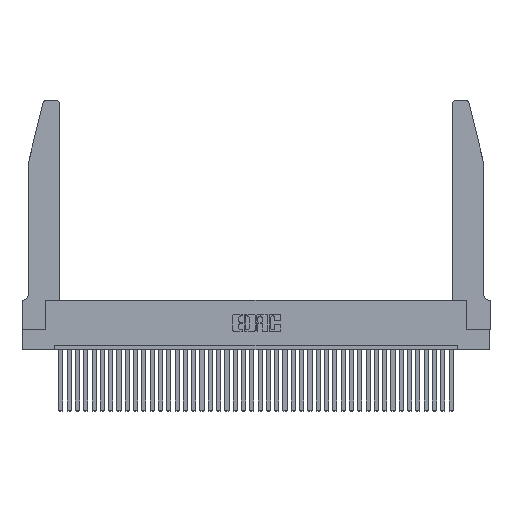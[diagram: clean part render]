
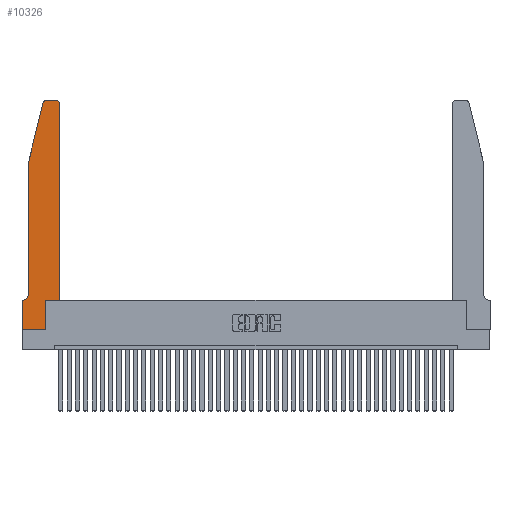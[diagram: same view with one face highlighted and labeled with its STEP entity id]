
A CAD part, top view. The second image highlights one B-rep face of the part: STEP entity #10326.
In plain terms, the highlighted planar face has unit normal (0, 0, 1).
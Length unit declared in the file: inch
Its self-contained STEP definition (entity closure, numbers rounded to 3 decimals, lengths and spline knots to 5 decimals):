
#589 = VERTEX_POINT ( 'NONE', #13890 ) ;
#645 = EDGE_CURVE ( 'NONE', #35161, #6498, #15695, .T. ) ;
#1042 = DIRECTION ( 'NONE',  ( 0., 1., 0. ) ) ;
#1490 = CARTESIAN_POINT ( 'NONE',  ( 0.4205, 2.75, 0.37 ) ) ;
#2235 = ORIENTED_EDGE ( 'NONE', *, *, #22283, .T. ) ;
#3429 = CIRCLE ( 'NONE', #34982, 0.03 ) ;
#4097 = VECTOR ( 'NONE', #7911, 39.37008 ) ;
#4209 = CARTESIAN_POINT ( 'NONE',  ( 0.4505, 0.35, 0.37 ) ) ;
#4305 = CARTESIAN_POINT ( 'NONE',  ( 0.0755, 2., 0.37 ) ) ;
#4544 = VECTOR ( 'NONE', #25176, 39.37008 ) ;
#4621 = LINE ( 'NONE', #5936, #9908 ) ;
#4705 = DIRECTION ( 'NONE',  ( 0., -1., 0. ) ) ;
#4820 = CARTESIAN_POINT ( 'NONE',  ( 0.2865, 0.35, 0.37 ) ) ;
#5300 = EDGE_CURVE ( 'NONE', #589, #15659, #29357, .T. ) ;
#5936 = CARTESIAN_POINT ( 'NONE',  ( 0.2605, 2.75, 0.37 ) ) ;
#6114 = CARTESIAN_POINT ( 'NONE',  ( 0., 0., 0.37 ) ) ;
#6163 = CARTESIAN_POINT ( 'NONE',  ( 0.284, 2.75, 0.37 ) ) ;
#6392 = EDGE_CURVE ( 'NONE', #20870, #37852, #35029, .T. ) ;
#6498 = VERTEX_POINT ( 'NONE', #14295 ) ;
#6623 = VECTOR ( 'NONE', #18837, 39.37008 ) ;
#7006 = VECTOR ( 'NONE', #1042, 39.37008 ) ;
#7141 = DIRECTION ( 'NONE',  ( 1., 0., 0. ) ) ;
#7183 = CARTESIAN_POINT ( 'NONE',  ( 0.0755, 0.35, 0.37 ) ) ;
#7505 = CARTESIAN_POINT ( 'NONE',  ( 0.0755, 2., 0.37 ) ) ;
#7640 = DIRECTION ( 'NONE',  ( -0.239, -0.971, 0. ) ) ;
#7911 = DIRECTION ( 'NONE',  ( 0., -1., 0. ) ) ;
#7989 = DIRECTION ( 'NONE',  ( 1., 0., 0. ) ) ;
#8179 = CARTESIAN_POINT ( 'NONE',  ( 0., 0.35, 0.37 ) ) ;
#8869 = EDGE_CURVE ( 'NONE', #38321, #37505, #3429, .T. ) ;
#8911 = DIRECTION ( 'NONE',  ( -1., 0., 0. ) ) ;
#9540 = LINE ( 'NONE', #6114, #6623 ) ;
#9835 = ORIENTED_EDGE ( 'NONE', *, *, #6392, .T. ) ;
#9908 = VECTOR ( 'NONE', #8911, 39.37008 ) ;
#10326 = ADVANCED_FACE ( 'NONE', ( #18311 ), #38948, .T. ) ;
#11363 = ORIENTED_EDGE ( 'NONE', *, *, #24480, .T. ) ;
#11389 = CARTESIAN_POINT ( 'NONE',  ( 0., 0., 0.37 ) ) ;
#11630 = CARTESIAN_POINT ( 'NONE',  ( 0., 0., 0.37 ) ) ;
#12373 = DIRECTION ( 'NONE',  ( -1., 0., 0. ) ) ;
#13304 = VECTOR ( 'NONE', #4705, 39.37008 ) ;
#13830 = CARTESIAN_POINT ( 'NONE',  ( 0.4505, 2.72, 0.37 ) ) ;
#13890 = CARTESIAN_POINT ( 'NONE',  ( 0.0755, 0.42, 0.37 ) ) ;
#14129 = DIRECTION ( 'NONE',  ( 1., 0., 0. ) ) ;
#14295 = CARTESIAN_POINT ( 'NONE',  ( 0.4505, 0.35, 0.37 ) ) ;
#14381 = DIRECTION ( 'NONE',  ( 0., 0., 1. ) ) ;
#15659 = VERTEX_POINT ( 'NONE', #33904 ) ;
#15695 = LINE ( 'NONE', #4209, #39764 ) ;
#16144 = CARTESIAN_POINT ( 'NONE',  ( 0.2865, 0.35, 0.37 ) ) ;
#17156 = DIRECTION ( 'NONE',  ( 1., 0., 0. ) ) ;
#17570 = ORIENTED_EDGE ( 'NONE', *, *, #8869, .T. ) ;
#17880 = ORIENTED_EDGE ( 'NONE', *, *, #645, .T. ) ;
#18311 = FACE_OUTER_BOUND ( 'NONE', #35953, .T. ) ;
#18477 = AXIS2_PLACEMENT_3D ( 'NONE', #8179, #14381, #14129 ) ;
#18837 = DIRECTION ( 'NONE',  ( 1., 0., 0. ) ) ;
#19329 = EDGE_CURVE ( 'NONE', #37852, #38331, #9540, .T. ) ;
#19630 = DIRECTION ( 'NONE',  ( -1., 0., 0. ) ) ;
#19661 = ORIENTED_EDGE ( 'NONE', *, *, #22123, .T. ) ;
#19864 = CARTESIAN_POINT ( 'NONE',  ( 0., 0.35, 0.37 ) ) ;
#20043 = LINE ( 'NONE', #34841, #7006 ) ;
#20467 = VECTOR ( 'NONE', #7640, 39.37008 ) ;
#20529 = DIRECTION ( 'NONE',  ( 0., 0., 1. ) ) ;
#20870 = VERTEX_POINT ( 'NONE', #19864 ) ;
#21017 = EDGE_CURVE ( 'NONE', #28596, #33190, #23920, .T. ) ;
#21242 = EDGE_CURVE ( 'NONE', #6498, #28596, #20043, .T. ) ;
#21863 = CARTESIAN_POINT ( 'NONE',  ( 0.0055, 0.42, 0.37 ) ) ;
#21864 = CARTESIAN_POINT ( 'NONE',  ( 0.0755, 2., 0.37 ) ) ;
#22123 = EDGE_CURVE ( 'NONE', #26755, #589, #32594, .T. ) ;
#22283 = EDGE_CURVE ( 'NONE', #37505, #26755, #29636, .T. ) ;
#23566 = DIRECTION ( 'NONE',  ( 0., 0., 1. ) ) ;
#23688 = CARTESIAN_POINT ( 'NONE',  ( 0.284, 2.72, 0.37 ) ) ;
#23920 = CIRCLE ( 'NONE', #24171, 0.03 ) ;
#24171 = AXIS2_PLACEMENT_3D ( 'NONE', #32954, #20529, #17156 ) ;
#24480 = EDGE_CURVE ( 'NONE', #15659, #20870, #31365, .T. ) ;
#24566 = DIRECTION ( 'NONE',  ( 0., 0., -1. ) ) ;
#25176 = DIRECTION ( 'NONE',  ( 0., 1., 0. ) ) ;
#26254 = ORIENTED_EDGE ( 'NONE', *, *, #30677, .T. ) ;
#26593 = EDGE_CURVE ( 'NONE', #38331, #35161, #30578, .T. ) ;
#26755 = VERTEX_POINT ( 'NONE', #21864 ) ;
#27018 = ORIENTED_EDGE ( 'NONE', *, *, #21242, .T. ) ;
#28596 = VERTEX_POINT ( 'NONE', #13830 ) ;
#28714 = ORIENTED_EDGE ( 'NONE', *, *, #21017, .T. ) ;
#29357 = CIRCLE ( 'NONE', #31567, 0.07 ) ;
#29636 = LINE ( 'NONE', #7505, #20467 ) ;
#29761 = ORIENTED_EDGE ( 'NONE', *, *, #19329, .T. ) ;
#30578 = LINE ( 'NONE', #16144, #4544 ) ;
#30677 = EDGE_CURVE ( 'NONE', #33190, #38321, #4621, .T. ) ;
#31365 = LINE ( 'NONE', #7183, #38596 ) ;
#31567 = AXIS2_PLACEMENT_3D ( 'NONE', #21863, #24566, #12373 ) ;
#32594 = LINE ( 'NONE', #4305, #4097 ) ;
#32954 = CARTESIAN_POINT ( 'NONE',  ( 0.4205, 2.72, 0.37 ) ) ;
#33190 = VERTEX_POINT ( 'NONE', #1490 ) ;
#33364 = ORIENTED_EDGE ( 'NONE', *, *, #5300, .T. ) ;
#33749 = ORIENTED_EDGE ( 'NONE', *, *, #26593, .T. ) ;
#33904 = CARTESIAN_POINT ( 'NONE',  ( 0.0055, 0.35, 0.37 ) ) ;
#34841 = CARTESIAN_POINT ( 'NONE',  ( 0.4505, 0.35, 0.37 ) ) ;
#34982 = AXIS2_PLACEMENT_3D ( 'NONE', #23688, #23566, #7989 ) ;
#35029 = LINE ( 'NONE', #11389, #13304 ) ;
#35161 = VERTEX_POINT ( 'NONE', #4820 ) ;
#35273 = CARTESIAN_POINT ( 'NONE',  ( 0.25487, 2.72718, 0.37 ) ) ;
#35953 = EDGE_LOOP ( 'NONE', ( #26254, #17570, #2235, #19661, #33364, #11363, #9835, #29761, #33749, #17880, #27018, #28714 ) ) ;
#36792 = CARTESIAN_POINT ( 'NONE',  ( 0.2865, 0., 0.37 ) ) ;
#37505 = VERTEX_POINT ( 'NONE', #35273 ) ;
#37852 = VERTEX_POINT ( 'NONE', #11630 ) ;
#38321 = VERTEX_POINT ( 'NONE', #6163 ) ;
#38331 = VERTEX_POINT ( 'NONE', #36792 ) ;
#38596 = VECTOR ( 'NONE', #19630, 39.37008 ) ;
#38948 = PLANE ( 'NONE',  #18477 ) ;
#39764 = VECTOR ( 'NONE', #7141, 39.37008 ) ;
